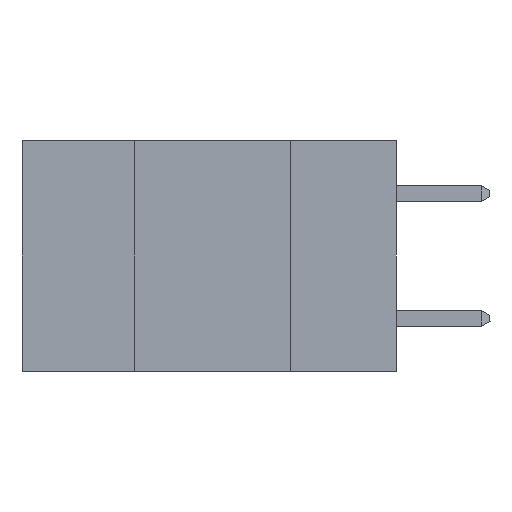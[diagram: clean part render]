
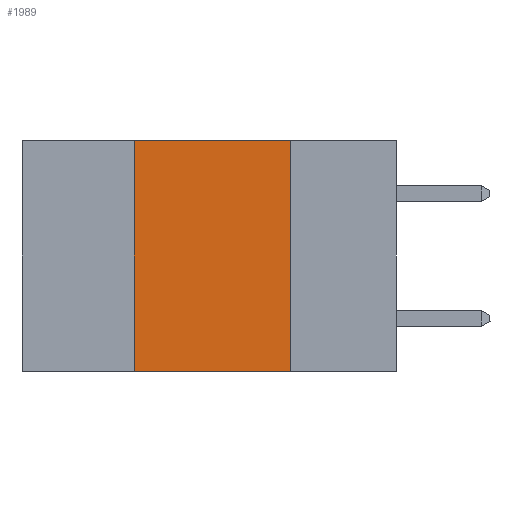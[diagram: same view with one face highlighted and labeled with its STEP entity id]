
A CAD part, left-side view. The second image highlights one B-rep face of the part: STEP entity #1989.
In plain terms, the highlighted planar face has unit normal (-1, 0, 0).
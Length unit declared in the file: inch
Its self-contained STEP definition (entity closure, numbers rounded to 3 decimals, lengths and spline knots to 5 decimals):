
#74 = DIRECTION ( 'NONE',  ( 0., -1., 0. ) ) ;
#158 = VERTEX_POINT ( 'NONE', #4595 ) ;
#208 = EDGE_CURVE ( 'NONE', #3925, #8543, #4017, .T. ) ;
#304 = CARTESIAN_POINT ( 'NONE',  ( 0., 0.6, 0. ) ) ;
#509 = VERTEX_POINT ( 'NONE', #2249 ) ;
#923 = VECTOR ( 'NONE', #2736, 39.37008 ) ;
#953 = CARTESIAN_POINT ( 'NONE',  ( 0., 0.42, 0. ) ) ;
#1075 = EDGE_CURVE ( 'NONE', #158, #509, #2672, .T. ) ;
#1200 = CARTESIAN_POINT ( 'NONE',  ( 0., 0.42, -0.37 ) ) ;
#1239 = LINE ( 'NONE', #6554, #6203 ) ;
#1503 = DIRECTION ( 'NONE',  ( 0., -1., 0. ) ) ;
#1572 = CARTESIAN_POINT ( 'NONE',  ( 0., 0.6, 0. ) ) ;
#1835 = ORIENTED_EDGE ( 'NONE', *, *, #208, .F. ) ;
#1989 = ADVANCED_FACE ( 'NONE', ( #9146 ), #2711, .F. ) ;
#2249 = CARTESIAN_POINT ( 'NONE',  ( 0., 0.17, -0.37 ) ) ;
#2410 = CARTESIAN_POINT ( 'NONE',  ( 0., 0.17, -0.37 ) ) ;
#2672 = LINE ( 'NONE', #2410, #923 ) ;
#2711 = PLANE ( 'NONE',  #5469 ) ;
#2736 = DIRECTION ( 'NONE',  ( 0., 0., -1. ) ) ;
#2860 = ORIENTED_EDGE ( 'NONE', *, *, #3007, .T. ) ;
#3007 = EDGE_CURVE ( 'NONE', #3925, #509, #1239, .T. ) ;
#3277 = ORIENTED_EDGE ( 'NONE', *, *, #1075, .F. ) ;
#3778 = CARTESIAN_POINT ( 'NONE',  ( 0., 0.42, -0.37 ) ) ;
#3925 = VERTEX_POINT ( 'NONE', #1200 ) ;
#4017 = LINE ( 'NONE', #3778, #7352 ) ;
#4595 = CARTESIAN_POINT ( 'NONE',  ( 0., 0.17, 0. ) ) ;
#5057 = DIRECTION ( 'NONE',  ( 1., 0., 0. ) ) ;
#5469 = AXIS2_PLACEMENT_3D ( 'NONE', #304, #5057, #8197 ) ;
#6203 = VECTOR ( 'NONE', #74, 39.37008 ) ;
#6465 = EDGE_CURVE ( 'NONE', #8543, #158, #8896, .T. ) ;
#6554 = CARTESIAN_POINT ( 'NONE',  ( 0., 0.6, -0.37 ) ) ;
#6878 = DIRECTION ( 'NONE',  ( 0., 0., 1. ) ) ;
#7352 = VECTOR ( 'NONE', #6878, 39.37008 ) ;
#7580 = ORIENTED_EDGE ( 'NONE', *, *, #6465, .F. ) ;
#7817 = VECTOR ( 'NONE', #1503, 39.37008 ) ;
#8197 = DIRECTION ( 'NONE',  ( 0., 0., -1. ) ) ;
#8543 = VERTEX_POINT ( 'NONE', #953 ) ;
#8595 = EDGE_LOOP ( 'NONE', ( #3277, #7580, #1835, #2860 ) ) ;
#8896 = LINE ( 'NONE', #1572, #7817 ) ;
#9146 = FACE_OUTER_BOUND ( 'NONE', #8595, .T. ) ;
